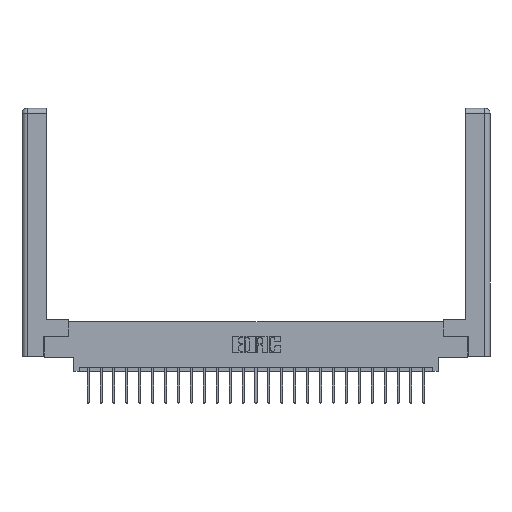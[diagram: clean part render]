
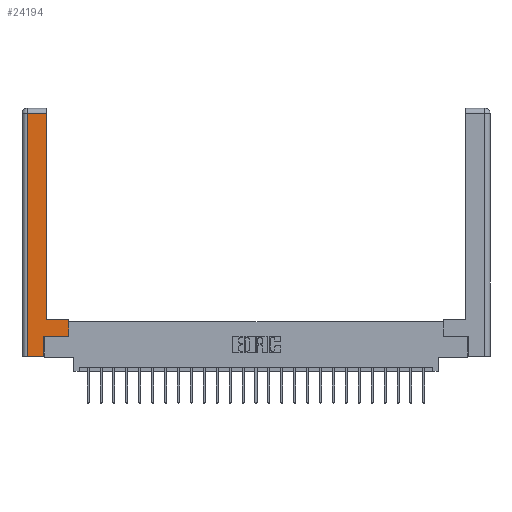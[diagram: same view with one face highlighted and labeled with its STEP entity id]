
A CAD part, top view. The second image highlights one B-rep face of the part: STEP entity #24194.
In plain terms, the highlighted planar face has unit normal (0, 0, 1).
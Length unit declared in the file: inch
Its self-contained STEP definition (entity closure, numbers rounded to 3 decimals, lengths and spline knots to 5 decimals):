
#280 = VERTEX_POINT ( 'NONE', #24319 ) ;
#402 = CARTESIAN_POINT ( 'NONE',  ( 0.565, 0.245, 0. ) ) ;
#438 = CARTESIAN_POINT ( 'NONE',  ( 0.295, 3., 0. ) ) ;
#514 = DIRECTION ( 'NONE',  ( 0., -1., 0. ) ) ;
#583 = FACE_OUTER_BOUND ( 'NONE', #20225, .T. ) ;
#833 = VERTEX_POINT ( 'NONE', #17062 ) ;
#1492 = LINE ( 'NONE', #402, #21940 ) ;
#2119 = VERTEX_POINT ( 'NONE', #24417 ) ;
#2214 = DIRECTION ( 'NONE',  ( -1., 0., 0. ) ) ;
#2560 = ORIENTED_EDGE ( 'NONE', *, *, #24509, .T. ) ;
#2651 = EDGE_CURVE ( 'NONE', #280, #2119, #11394, .T. ) ;
#2663 = AXIS2_PLACEMENT_3D ( 'NONE', #25333, #3286, #11132 ) ;
#3241 = ORIENTED_EDGE ( 'NONE', *, *, #5345, .T. ) ;
#3286 = DIRECTION ( 'NONE',  ( 0., 0., -1. ) ) ;
#3671 = EDGE_CURVE ( 'NONE', #5470, #21950, #19455, .T. ) ;
#4192 = VECTOR ( 'NONE', #6287, 39.37008 ) ;
#4377 = CARTESIAN_POINT ( 'NONE',  ( 0.0615, 0., 0. ) ) ;
#4808 = LINE ( 'NONE', #16265, #4192 ) ;
#5116 = LINE ( 'NONE', #438, #6368 ) ;
#5345 = EDGE_CURVE ( 'NONE', #18296, #16896, #5116, .T. ) ;
#5427 = EDGE_CURVE ( 'NONE', #833, #12773, #19714, .T. ) ;
#5470 = VERTEX_POINT ( 'NONE', #13004 ) ;
#6099 = CARTESIAN_POINT ( 'NONE',  ( 0.265, 0.245, 0. ) ) ;
#6287 = DIRECTION ( 'NONE',  ( -1., 0., 0. ) ) ;
#6368 = VECTOR ( 'NONE', #8258, 39.37008 ) ;
#8236 = LINE ( 'NONE', #22323, #8748 ) ;
#8258 = DIRECTION ( 'NONE',  ( 0., 1., 0. ) ) ;
#8748 = VECTOR ( 'NONE', #2214, 39.37008 ) ;
#8764 = LINE ( 'NONE', #11739, #24002 ) ;
#9184 = CARTESIAN_POINT ( 'NONE',  ( 0.565, 0.45, 0. ) ) ;
#9673 = DIRECTION ( 'NONE',  ( 1., 0., 0. ) ) ;
#9887 = ORIENTED_EDGE ( 'NONE', *, *, #11002, .T. ) ;
#10686 = ORIENTED_EDGE ( 'NONE', *, *, #3671, .T. ) ;
#11002 = EDGE_CURVE ( 'NONE', #16896, #833, #4808, .T. ) ;
#11132 = DIRECTION ( 'NONE',  ( -1., 0., 0. ) ) ;
#11394 = LINE ( 'NONE', #6099, #13591 ) ;
#11455 = ORIENTED_EDGE ( 'NONE', *, *, #2651, .T. ) ;
#11642 = VECTOR ( 'NONE', #18877, 39.37008 ) ;
#11739 = CARTESIAN_POINT ( 'NONE',  ( 0.265, 0., 0. ) ) ;
#12773 = VERTEX_POINT ( 'NONE', #20774 ) ;
#13004 = CARTESIAN_POINT ( 'NONE',  ( 0.565, 0.245, 0. ) ) ;
#13591 = VECTOR ( 'NONE', #20222, 39.37008 ) ;
#14851 = ORIENTED_EDGE ( 'NONE', *, *, #5427, .T. ) ;
#16265 = CARTESIAN_POINT ( 'NONE',  ( 0.0615, 2.94, 0. ) ) ;
#16567 = CARTESIAN_POINT ( 'NONE',  ( 0.565, 0.45, 0. ) ) ;
#16646 = EDGE_CURVE ( 'NONE', #12773, #280, #8764, .T. ) ;
#16896 = VERTEX_POINT ( 'NONE', #18597 ) ;
#17062 = CARTESIAN_POINT ( 'NONE',  ( 0.0615, 2.94, 0. ) ) ;
#17158 = ORIENTED_EDGE ( 'NONE', *, *, #16646, .T. ) ;
#17882 = DIRECTION ( 'NONE',  ( 1., 0., 0. ) ) ;
#18296 = VERTEX_POINT ( 'NONE', #21261 ) ;
#18597 = CARTESIAN_POINT ( 'NONE',  ( 0.295, 2.94, 0. ) ) ;
#18877 = DIRECTION ( 'NONE',  ( 0., 1., 0. ) ) ;
#19319 = PLANE ( 'NONE',  #2663 ) ;
#19455 = LINE ( 'NONE', #16567, #11642 ) ;
#19714 = LINE ( 'NONE', #4377, #21870 ) ;
#20222 = DIRECTION ( 'NONE',  ( 0., 1., 0. ) ) ;
#20225 = EDGE_LOOP ( 'NONE', ( #3241, #9887, #14851, #17158, #11455, #21074, #10686, #2560 ) ) ;
#20774 = CARTESIAN_POINT ( 'NONE',  ( 0.0615, 0., 0. ) ) ;
#21074 = ORIENTED_EDGE ( 'NONE', *, *, #24063, .T. ) ;
#21261 = CARTESIAN_POINT ( 'NONE',  ( 0.295, 0.45, 0. ) ) ;
#21870 = VECTOR ( 'NONE', #514, 39.37008 ) ;
#21940 = VECTOR ( 'NONE', #17882, 39.37008 ) ;
#21950 = VERTEX_POINT ( 'NONE', #9184 ) ;
#22323 = CARTESIAN_POINT ( 'NONE',  ( 0.295, 0.45, 0. ) ) ;
#24002 = VECTOR ( 'NONE', #9673, 39.37008 ) ;
#24063 = EDGE_CURVE ( 'NONE', #2119, #5470, #1492, .T. ) ;
#24194 = ADVANCED_FACE ( 'NONE', ( #583 ), #19319, .F. ) ;
#24319 = CARTESIAN_POINT ( 'NONE',  ( 0.265, 0., 0. ) ) ;
#24417 = CARTESIAN_POINT ( 'NONE',  ( 0.265, 0.245, 0. ) ) ;
#24509 = EDGE_CURVE ( 'NONE', #21950, #18296, #8236, .T. ) ;
#25333 = CARTESIAN_POINT ( 'NONE',  ( 0., 0., 0. ) ) ;
